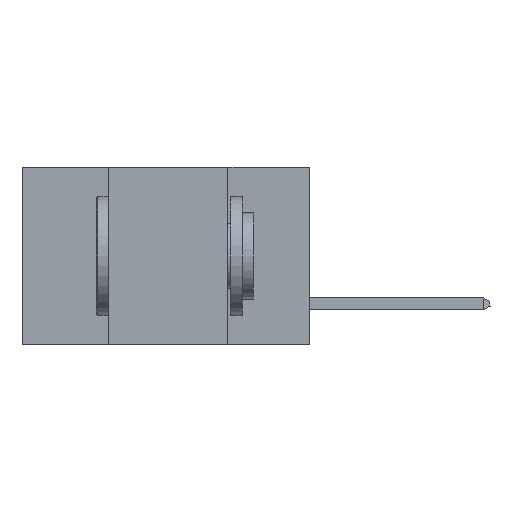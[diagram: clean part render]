
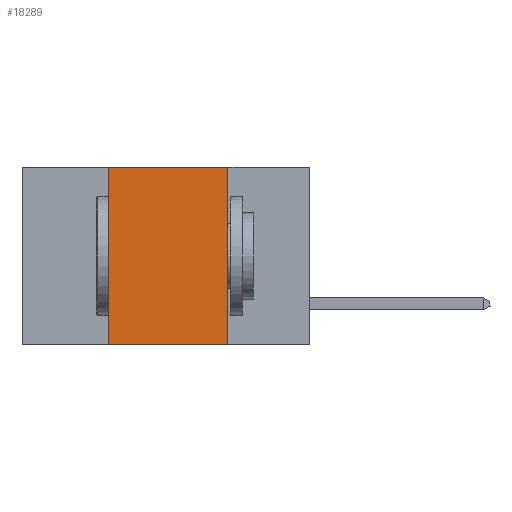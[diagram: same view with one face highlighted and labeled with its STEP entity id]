
A CAD part, left-side view. The second image highlights one B-rep face of the part: STEP entity #18289.
In plain terms, the highlighted planar face has unit normal (-1, 0, 0).
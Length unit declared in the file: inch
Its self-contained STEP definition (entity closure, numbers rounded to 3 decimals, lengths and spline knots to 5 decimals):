
#605 = VECTOR ( 'NONE', #9592, 39.37008 ) ;
#634 = ORIENTED_EDGE ( 'NONE', *, *, #1476, .F. ) ;
#869 = VERTEX_POINT ( 'NONE', #4396 ) ;
#1476 = EDGE_CURVE ( 'NONE', #869, #17643, #4548, .T. ) ;
#1637 = EDGE_CURVE ( 'NONE', #11317, #7954, #14513, .T. ) ;
#1737 = CARTESIAN_POINT ( 'NONE',  ( 0., 0.42, 0. ) ) ;
#1759 = DIRECTION ( 'NONE',  ( 0., 0., -1. ) ) ;
#1816 = CARTESIAN_POINT ( 'NONE',  ( 0., 0.17, -0.37 ) ) ;
#2926 = CARTESIAN_POINT ( 'NONE',  ( 0., 0.17, 0. ) ) ;
#2944 = EDGE_CURVE ( 'NONE', #17643, #7954, #12280, .T. ) ;
#3684 = DIRECTION ( 'NONE',  ( 0., 0., -1. ) ) ;
#3752 = LINE ( 'NONE', #1737, #605 ) ;
#4282 = FACE_OUTER_BOUND ( 'NONE', #6113, .T. ) ;
#4396 = CARTESIAN_POINT ( 'NONE',  ( 0., 0.42, 0. ) ) ;
#4548 = LINE ( 'NONE', #7391, #13290 ) ;
#5588 = CARTESIAN_POINT ( 'NONE',  ( 0., 0.42, -0.37 ) ) ;
#5662 = ORIENTED_EDGE ( 'NONE', *, *, #9401, .F. ) ;
#6113 = EDGE_LOOP ( 'NONE', ( #7870, #634, #5662, #15632 ) ) ;
#7391 = CARTESIAN_POINT ( 'NONE',  ( 0., 0.6, 0. ) ) ;
#7704 = VECTOR ( 'NONE', #9448, 39.37008 ) ;
#7870 = ORIENTED_EDGE ( 'NONE', *, *, #2944, .F. ) ;
#7954 = VERTEX_POINT ( 'NONE', #1816 ) ;
#9401 = EDGE_CURVE ( 'NONE', #11317, #869, #3752, .T. ) ;
#9448 = DIRECTION ( 'NONE',  ( 0., -1., 0. ) ) ;
#9479 = PLANE ( 'NONE',  #10047 ) ;
#9592 = DIRECTION ( 'NONE',  ( 0., 0., 1. ) ) ;
#10047 = AXIS2_PLACEMENT_3D ( 'NONE', #18966, #15738, #1759 ) ;
#11317 = VERTEX_POINT ( 'NONE', #5588 ) ;
#12280 = LINE ( 'NONE', #19118, #18044 ) ;
#13290 = VECTOR ( 'NONE', #16525, 39.37008 ) ;
#14116 = CARTESIAN_POINT ( 'NONE',  ( 0., 0.6, -0.37 ) ) ;
#14513 = LINE ( 'NONE', #14116, #7704 ) ;
#15632 = ORIENTED_EDGE ( 'NONE', *, *, #1637, .T. ) ;
#15738 = DIRECTION ( 'NONE',  ( 1., 0., 0. ) ) ;
#16525 = DIRECTION ( 'NONE',  ( 0., -1., 0. ) ) ;
#17643 = VERTEX_POINT ( 'NONE', #2926 ) ;
#18044 = VECTOR ( 'NONE', #3684, 39.37008 ) ;
#18289 = ADVANCED_FACE ( 'NONE', ( #4282 ), #9479, .F. ) ;
#18966 = CARTESIAN_POINT ( 'NONE',  ( 0., 0.6, 0. ) ) ;
#19118 = CARTESIAN_POINT ( 'NONE',  ( 0., 0.17, 0. ) ) ;
